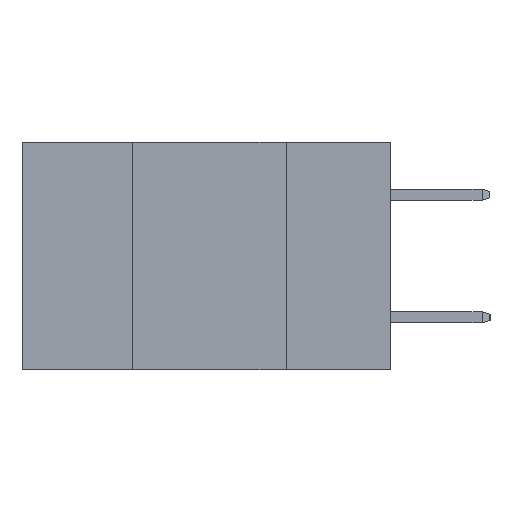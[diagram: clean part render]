
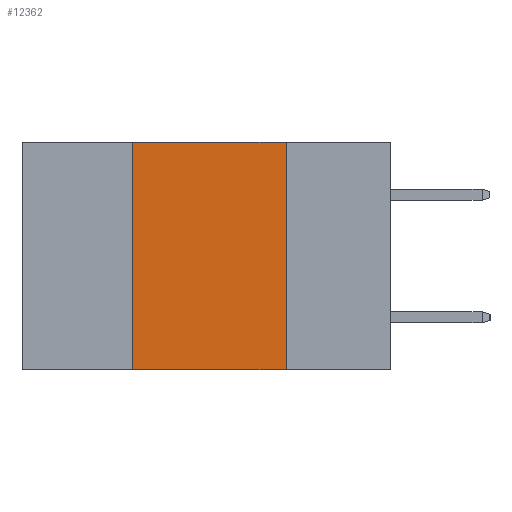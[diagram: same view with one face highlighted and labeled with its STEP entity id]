
A CAD part, left-side view. The second image highlights one B-rep face of the part: STEP entity #12362.
In plain terms, the highlighted planar face has unit normal (-1, 0, 0).
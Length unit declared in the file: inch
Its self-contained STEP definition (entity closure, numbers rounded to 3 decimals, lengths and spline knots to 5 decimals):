
#540 = EDGE_CURVE ( 'NONE', #2464, #5876, #11485, .T. ) ;
#937 = ORIENTED_EDGE ( 'NONE', *, *, #8376, .F. ) ;
#981 = PLANE ( 'NONE',  #12899 ) ;
#1054 = CARTESIAN_POINT ( 'NONE',  ( 0., 0.6, -0.37 ) ) ;
#1965 = ORIENTED_EDGE ( 'NONE', *, *, #3425, .T. ) ;
#2140 = CARTESIAN_POINT ( 'NONE',  ( 0., 0.42, 0. ) ) ;
#2464 = VERTEX_POINT ( 'NONE', #8240 ) ;
#2840 = EDGE_LOOP ( 'NONE', ( #12165, #937, #11755, #1965 ) ) ;
#2931 = LINE ( 'NONE', #11302, #4062 ) ;
#3117 = DIRECTION ( 'NONE',  ( 1., 0., 0. ) ) ;
#3425 = EDGE_CURVE ( 'NONE', #6362, #5876, #11736, .T. ) ;
#3464 = DIRECTION ( 'NONE',  ( 0., 0., -1. ) ) ;
#4062 = VECTOR ( 'NONE', #10138, 39.37008 ) ;
#4069 = CARTESIAN_POINT ( 'NONE',  ( 0., 0.6, 0. ) ) ;
#4989 = DIRECTION ( 'NONE',  ( 0., 0., 1. ) ) ;
#5876 = VERTEX_POINT ( 'NONE', #10240 ) ;
#6263 = DIRECTION ( 'NONE',  ( 0., -1., 0. ) ) ;
#6362 = VERTEX_POINT ( 'NONE', #12075 ) ;
#6597 = VECTOR ( 'NONE', #4989, 39.37008 ) ;
#6696 = CARTESIAN_POINT ( 'NONE',  ( 0., 0.17, 0. ) ) ;
#7184 = EDGE_CURVE ( 'NONE', #6362, #13209, #7252, .T. ) ;
#7252 = LINE ( 'NONE', #8158, #6597 ) ;
#8158 = CARTESIAN_POINT ( 'NONE',  ( 0., 0.42, 0. ) ) ;
#8240 = CARTESIAN_POINT ( 'NONE',  ( 0., 0.17, 0. ) ) ;
#8376 = EDGE_CURVE ( 'NONE', #13209, #2464, #2931, .T. ) ;
#8608 = VECTOR ( 'NONE', #6263, 39.37008 ) ;
#10138 = DIRECTION ( 'NONE',  ( 0., -1., 0. ) ) ;
#10240 = CARTESIAN_POINT ( 'NONE',  ( 0., 0.17, -0.37 ) ) ;
#10627 = FACE_OUTER_BOUND ( 'NONE', #2840, .T. ) ;
#11302 = CARTESIAN_POINT ( 'NONE',  ( 0., 0.6, 0. ) ) ;
#11485 = LINE ( 'NONE', #6696, #12143 ) ;
#11736 = LINE ( 'NONE', #1054, #8608 ) ;
#11755 = ORIENTED_EDGE ( 'NONE', *, *, #7184, .F. ) ;
#12075 = CARTESIAN_POINT ( 'NONE',  ( 0., 0.42, -0.37 ) ) ;
#12143 = VECTOR ( 'NONE', #3464, 39.37008 ) ;
#12165 = ORIENTED_EDGE ( 'NONE', *, *, #540, .F. ) ;
#12362 = ADVANCED_FACE ( 'NONE', ( #10627 ), #981, .F. ) ;
#12899 = AXIS2_PLACEMENT_3D ( 'NONE', #4069, #3117, #13465 ) ;
#13209 = VERTEX_POINT ( 'NONE', #2140 ) ;
#13465 = DIRECTION ( 'NONE',  ( 0., 0., -1. ) ) ;
